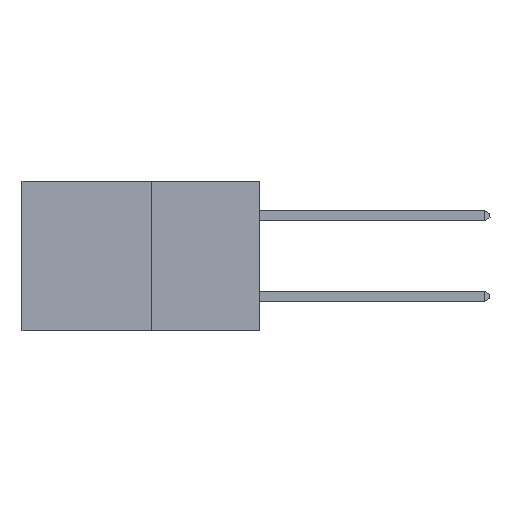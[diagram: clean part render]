
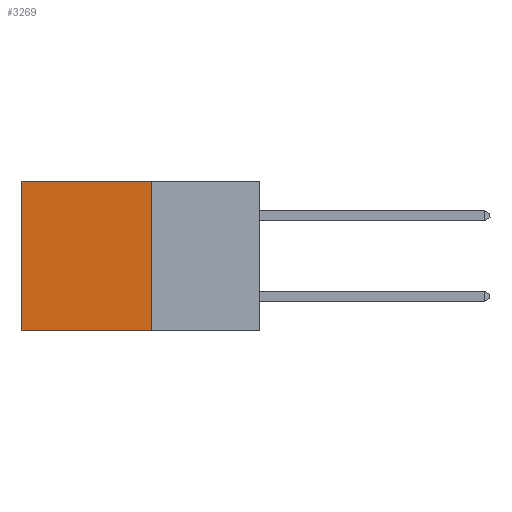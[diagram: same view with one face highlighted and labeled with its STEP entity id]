
A CAD part, left-side view. The second image highlights one B-rep face of the part: STEP entity #3269.
In plain terms, the highlighted planar face has unit normal (-1, 0, 0).
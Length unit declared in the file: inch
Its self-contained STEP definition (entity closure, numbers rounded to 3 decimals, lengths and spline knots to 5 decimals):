
#641 = VERTEX_POINT ( 'NONE', #4631 ) ;
#923 = CARTESIAN_POINT ( 'NONE',  ( 0.277, 0.59, -0.37 ) ) ;
#1055 = EDGE_CURVE ( 'NONE', #2546, #641, #1520, .T. ) ;
#1128 = DIRECTION ( 'NONE',  ( 0., 1., 0. ) ) ;
#1138 = CARTESIAN_POINT ( 'NONE',  ( 0.277, 0.59, 0. ) ) ;
#1520 = LINE ( 'NONE', #4128, #3122 ) ;
#1616 = VECTOR ( 'NONE', #1128, 39.37008 ) ;
#2164 = CARTESIAN_POINT ( 'NONE',  ( 0.277, 0.27, -0.37 ) ) ;
#2257 = FACE_OUTER_BOUND ( 'NONE', #3690, .T. ) ;
#2546 = VERTEX_POINT ( 'NONE', #6629 ) ;
#2562 = ORIENTED_EDGE ( 'NONE', *, *, #6491, .T. ) ;
#2608 = LINE ( 'NONE', #2707, #7108 ) ;
#2699 = PLANE ( 'NONE',  #6930 ) ;
#2707 = CARTESIAN_POINT ( 'NONE',  ( 0.277, 0.27, 0. ) ) ;
#2753 = ORIENTED_EDGE ( 'NONE', *, *, #6094, .F. ) ;
#2861 = DIRECTION ( 'NONE',  ( 1., 0., 0. ) ) ;
#3122 = VECTOR ( 'NONE', #4218, 39.37008 ) ;
#3214 = LINE ( 'NONE', #2164, #1616 ) ;
#3269 = ADVANCED_FACE ( 'NONE', ( #2257 ), #2699, .F. ) ;
#3690 = EDGE_LOOP ( 'NONE', ( #2562, #2753, #4350, #7403 ) ) ;
#4128 = CARTESIAN_POINT ( 'NONE',  ( 0.277, 0.27, -0.37 ) ) ;
#4212 = VERTEX_POINT ( 'NONE', #1138 ) ;
#4218 = DIRECTION ( 'NONE',  ( 0., 0., -1. ) ) ;
#4350 = ORIENTED_EDGE ( 'NONE', *, *, #1055, .F. ) ;
#4477 = EDGE_CURVE ( 'NONE', #2546, #4212, #2608, .T. ) ;
#4631 = CARTESIAN_POINT ( 'NONE',  ( 0.277, 0.27, -0.37 ) ) ;
#4858 = CARTESIAN_POINT ( 'NONE',  ( 0.277, 0.27, -0.37 ) ) ;
#5172 = VERTEX_POINT ( 'NONE', #923 ) ;
#5259 = CARTESIAN_POINT ( 'NONE',  ( 0.277, 0.59, -0.37 ) ) ;
#5523 = DIRECTION ( 'NONE',  ( 0., 0., -1. ) ) ;
#5565 = LINE ( 'NONE', #5259, #6711 ) ;
#6094 = EDGE_CURVE ( 'NONE', #641, #5172, #3214, .T. ) ;
#6491 = EDGE_CURVE ( 'NONE', #4212, #5172, #5565, .T. ) ;
#6629 = CARTESIAN_POINT ( 'NONE',  ( 0.277, 0.27, 0. ) ) ;
#6711 = VECTOR ( 'NONE', #5523, 39.37008 ) ;
#6746 = DIRECTION ( 'NONE',  ( 0., 0., -1. ) ) ;
#6930 = AXIS2_PLACEMENT_3D ( 'NONE', #4858, #2861, #6746 ) ;
#7108 = VECTOR ( 'NONE', #7500, 39.37008 ) ;
#7403 = ORIENTED_EDGE ( 'NONE', *, *, #4477, .T. ) ;
#7500 = DIRECTION ( 'NONE',  ( 0., 1., 0. ) ) ;
